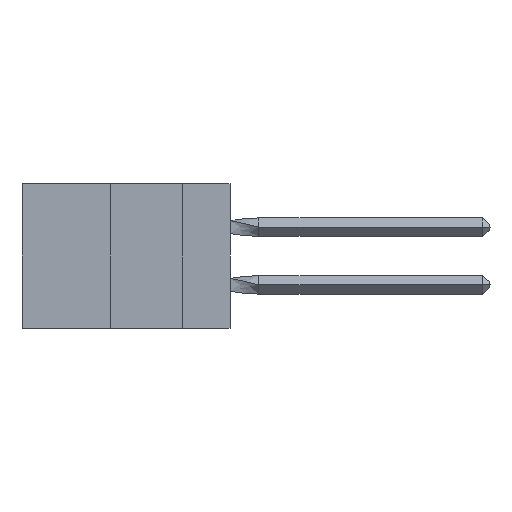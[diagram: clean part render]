
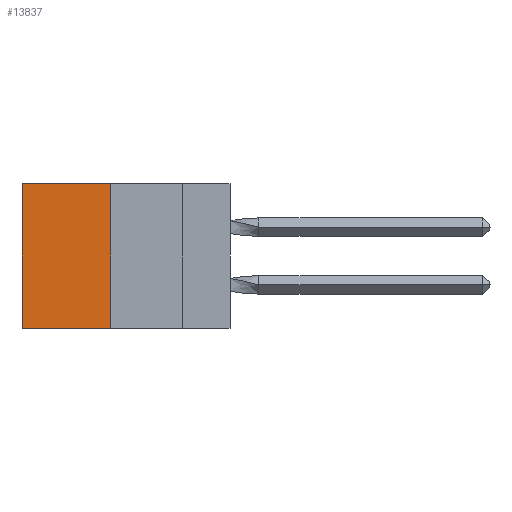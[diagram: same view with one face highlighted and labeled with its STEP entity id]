
A CAD part, left-side view. The second image highlights one B-rep face of the part: STEP entity #13837.
In plain terms, the highlighted planar face has unit normal (-1, 0, 0).
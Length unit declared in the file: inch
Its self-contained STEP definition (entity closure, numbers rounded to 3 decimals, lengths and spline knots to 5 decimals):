
#319 = ORIENTED_EDGE ( 'NONE', *, *, #16709, .F. ) ;
#650 = DIRECTION ( 'NONE',  ( 0., 0., -1. ) ) ;
#1201 = LINE ( 'NONE', #4692, #2457 ) ;
#1477 = LINE ( 'NONE', #4800, #11035 ) ;
#2457 = VECTOR ( 'NONE', #650, 39.37008 ) ;
#2680 = LINE ( 'NONE', #15405, #12052 ) ;
#2936 = VERTEX_POINT ( 'NONE', #3381 ) ;
#3381 = CARTESIAN_POINT ( 'NONE',  ( 0.305, 0.413, -0.5 ) ) ;
#4268 = VECTOR ( 'NONE', #8563, 39.37008 ) ;
#4562 = DIRECTION ( 'NONE',  ( 0., 0., -1. ) ) ;
#4692 = CARTESIAN_POINT ( 'NONE',  ( 0.305, 0.72, -0.5 ) ) ;
#4800 = CARTESIAN_POINT ( 'NONE',  ( 0.305, 0.413, -0.5 ) ) ;
#4972 = EDGE_LOOP ( 'NONE', ( #5424, #319, #8884, #7758 ) ) ;
#5424 = ORIENTED_EDGE ( 'NONE', *, *, #13227, .T. ) ;
#5838 = FACE_OUTER_BOUND ( 'NONE', #4972, .T. ) ;
#6360 = PLANE ( 'NONE',  #13148 ) ;
#6449 = VERTEX_POINT ( 'NONE', #8441 ) ;
#6753 = VERTEX_POINT ( 'NONE', #15011 ) ;
#7758 = ORIENTED_EDGE ( 'NONE', *, *, #12768, .T. ) ;
#8320 = LINE ( 'NONE', #13973, #4268 ) ;
#8441 = CARTESIAN_POINT ( 'NONE',  ( 0.305, 0.72, -0.5 ) ) ;
#8563 = DIRECTION ( 'NONE',  ( 0., 1., 0. ) ) ;
#8884 = ORIENTED_EDGE ( 'NONE', *, *, #11581, .F. ) ;
#9055 = DIRECTION ( 'NONE',  ( 0., 0., -1. ) ) ;
#11035 = VECTOR ( 'NONE', #4562, 39.37008 ) ;
#11581 = EDGE_CURVE ( 'NONE', #12334, #2936, #1477, .T. ) ;
#12052 = VECTOR ( 'NONE', #13966, 39.37008 ) ;
#12334 = VERTEX_POINT ( 'NONE', #14338 ) ;
#12768 = EDGE_CURVE ( 'NONE', #12334, #6753, #2680, .T. ) ;
#13035 = CARTESIAN_POINT ( 'NONE',  ( 0.305, 0.413, -0.5 ) ) ;
#13148 = AXIS2_PLACEMENT_3D ( 'NONE', #13035, #13266, #9055 ) ;
#13227 = EDGE_CURVE ( 'NONE', #6753, #6449, #1201, .T. ) ;
#13266 = DIRECTION ( 'NONE',  ( 1., 0., 0. ) ) ;
#13837 = ADVANCED_FACE ( 'NONE', ( #5838 ), #6360, .F. ) ;
#13966 = DIRECTION ( 'NONE',  ( 0., 1., 0. ) ) ;
#13973 = CARTESIAN_POINT ( 'NONE',  ( 0.305, 0.413, -0.5 ) ) ;
#14338 = CARTESIAN_POINT ( 'NONE',  ( 0.305, 0.413, 0. ) ) ;
#15011 = CARTESIAN_POINT ( 'NONE',  ( 0.305, 0.72, 0. ) ) ;
#15405 = CARTESIAN_POINT ( 'NONE',  ( 0.305, 0.413, 0. ) ) ;
#16709 = EDGE_CURVE ( 'NONE', #2936, #6449, #8320, .T. ) ;
